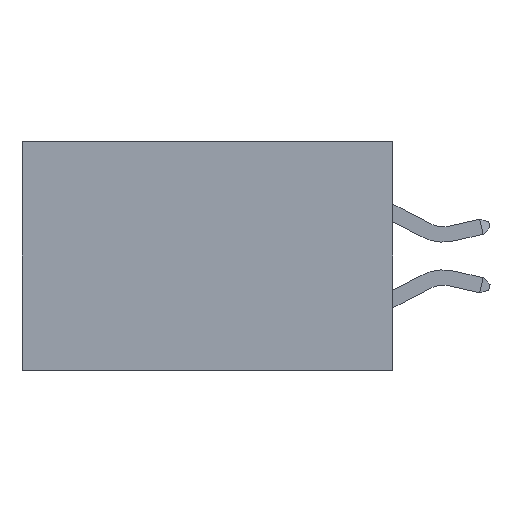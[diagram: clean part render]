
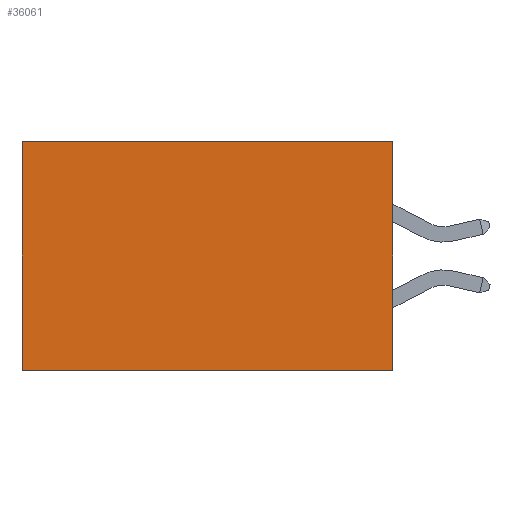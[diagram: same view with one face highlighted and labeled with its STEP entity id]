
A CAD part, left-side view. The second image highlights one B-rep face of the part: STEP entity #36061.
In plain terms, the highlighted planar face has unit normal (-1, 0, 0).
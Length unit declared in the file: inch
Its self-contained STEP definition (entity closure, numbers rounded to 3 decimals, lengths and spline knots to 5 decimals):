
#256 = EDGE_CURVE ( 'NONE', #23283, #8179, #33924, .T. ) ;
#362 = AXIS2_PLACEMENT_3D ( 'NONE', #35001, #14825, #38093 ) ;
#871 = ORIENTED_EDGE ( 'NONE', *, *, #256, .F. ) ;
#1992 = VECTOR ( 'NONE', #8593, 39.37008 ) ;
#7848 = CARTESIAN_POINT ( 'NONE',  ( 0.2875, 0., -0.37 ) ) ;
#8179 = VERTEX_POINT ( 'NONE', #16064 ) ;
#8593 = DIRECTION ( 'NONE',  ( 0., 1., 0. ) ) ;
#8648 = DIRECTION ( 'NONE',  ( 0., 1., 0. ) ) ;
#8781 = EDGE_CURVE ( 'NONE', #20355, #23283, #9076, .T. ) ;
#9076 = LINE ( 'NONE', #19312, #21722 ) ;
#10500 = CARTESIAN_POINT ( 'NONE',  ( 0.2875, 0., 0. ) ) ;
#11932 = VECTOR ( 'NONE', #8648, 39.37008 ) ;
#12339 = ORIENTED_EDGE ( 'NONE', *, *, #8781, .F. ) ;
#14396 = PLANE ( 'NONE',  #362 ) ;
#14796 = EDGE_CURVE ( 'NONE', #20355, #33856, #20861, .T. ) ;
#14825 = DIRECTION ( 'NONE',  ( 1., 0., 0. ) ) ;
#16064 = CARTESIAN_POINT ( 'NONE',  ( 0.2875, 0.6, -0.37 ) ) ;
#16247 = DIRECTION ( 'NONE',  ( 0., 0., -1. ) ) ;
#17107 = LINE ( 'NONE', #37741, #36989 ) ;
#19312 = CARTESIAN_POINT ( 'NONE',  ( 0.2875, 0., 0. ) ) ;
#20355 = VERTEX_POINT ( 'NONE', #10500 ) ;
#20861 = LINE ( 'NONE', #41738, #11932 ) ;
#21722 = VECTOR ( 'NONE', #16247, 39.37008 ) ;
#23283 = VERTEX_POINT ( 'NONE', #7848 ) ;
#23861 = EDGE_LOOP ( 'NONE', ( #36486, #871, #12339, #34994 ) ) ;
#26550 = EDGE_CURVE ( 'NONE', #33856, #8179, #17107, .T. ) ;
#28569 = FACE_OUTER_BOUND ( 'NONE', #23861, .T. ) ;
#31525 = CARTESIAN_POINT ( 'NONE',  ( 0.2875, 0.6, 0. ) ) ;
#31882 = CARTESIAN_POINT ( 'NONE',  ( 0.2875, 0., -0.37 ) ) ;
#33856 = VERTEX_POINT ( 'NONE', #31525 ) ;
#33924 = LINE ( 'NONE', #31882, #1992 ) ;
#33971 = DIRECTION ( 'NONE',  ( 0., 0., -1. ) ) ;
#34994 = ORIENTED_EDGE ( 'NONE', *, *, #14796, .T. ) ;
#35001 = CARTESIAN_POINT ( 'NONE',  ( 0.2875, 0., 0. ) ) ;
#36061 = ADVANCED_FACE ( 'NONE', ( #28569 ), #14396, .F. ) ;
#36486 = ORIENTED_EDGE ( 'NONE', *, *, #26550, .T. ) ;
#36989 = VECTOR ( 'NONE', #33971, 39.37008 ) ;
#37741 = CARTESIAN_POINT ( 'NONE',  ( 0.2875, 0.6, 0. ) ) ;
#38093 = DIRECTION ( 'NONE',  ( 0., 0., -1. ) ) ;
#41738 = CARTESIAN_POINT ( 'NONE',  ( 0.2875, 0., 0. ) ) ;
